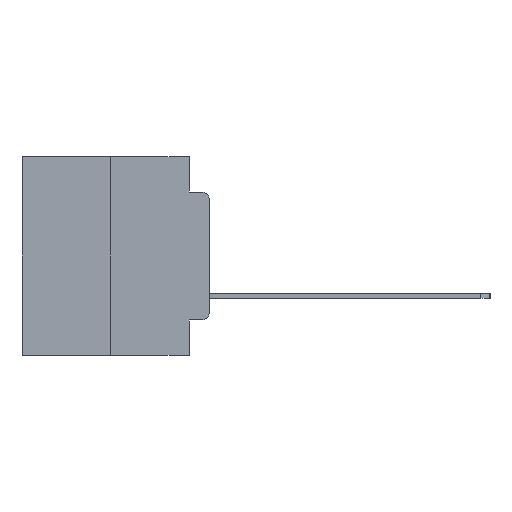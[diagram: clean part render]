
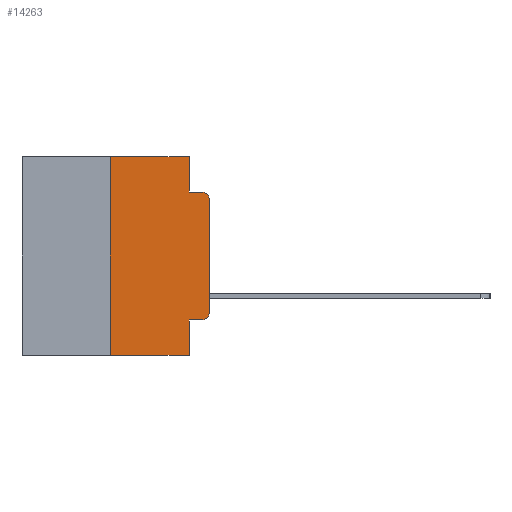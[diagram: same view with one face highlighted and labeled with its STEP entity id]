
A CAD part, left-side view. The second image highlights one B-rep face of the part: STEP entity #14263.
In plain terms, the highlighted planar face has unit normal (-1, 0, 0).
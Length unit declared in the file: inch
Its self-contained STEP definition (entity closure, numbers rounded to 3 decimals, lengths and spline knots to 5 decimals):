
#184 = CARTESIAN_POINT ( 'NONE',  ( 0., 0.051, -0.4115 ) ) ;
#255 = CARTESIAN_POINT ( 'NONE',  ( 0., 0.051, -0.5 ) ) ;
#302 = CARTESIAN_POINT ( 'NONE',  ( 0., 0.25, -0.5 ) ) ;
#664 = VERTEX_POINT ( 'NONE', #302 ) ;
#765 = DIRECTION ( 'NONE',  ( 0., 0., -1. ) ) ;
#1429 = CARTESIAN_POINT ( 'NONE',  ( 0., 0.25, 0. ) ) ;
#1545 = CIRCLE ( 'NONE', #26477, 0.02 ) ;
#1631 = CARTESIAN_POINT ( 'NONE',  ( 0., 0.25, 0. ) ) ;
#1742 = LINE ( 'NONE', #17916, #17604 ) ;
#2095 = VECTOR ( 'NONE', #19553, 39.37008 ) ;
#2428 = PLANE ( 'NONE',  #7140 ) ;
#3873 = CARTESIAN_POINT ( 'NONE',  ( 0., 0.02, -0.1085 ) ) ;
#4136 = VECTOR ( 'NONE', #13969, 39.37008 ) ;
#4396 = VERTEX_POINT ( 'NONE', #21142 ) ;
#4812 = VERTEX_POINT ( 'NONE', #255 ) ;
#5426 = CARTESIAN_POINT ( 'NONE',  ( 0., 0.473, -0.5 ) ) ;
#5463 = DIRECTION ( 'NONE',  ( 0., 0., -1. ) ) ;
#5525 = LINE ( 'NONE', #1429, #4136 ) ;
#6097 = DIRECTION ( 'NONE',  ( 0., 0., -1. ) ) ;
#6150 = VERTEX_POINT ( 'NONE', #8115 ) ;
#6629 = EDGE_CURVE ( 'NONE', #664, #4812, #7875, .T. ) ;
#6829 = DIRECTION ( 'NONE',  ( 0., 0., -1. ) ) ;
#7140 = AXIS2_PLACEMENT_3D ( 'NONE', #16870, #18857, #6829 ) ;
#7439 = EDGE_CURVE ( 'NONE', #664, #12577, #5525, .T. ) ;
#7503 = CARTESIAN_POINT ( 'NONE',  ( 0., 0.051, 0. ) ) ;
#7695 = EDGE_LOOP ( 'NONE', ( #23979, #17189, #19660, #12799, #21220, #23077, #20922, #14076, #24613, #19978 ) ) ;
#7875 = LINE ( 'NONE', #5426, #2095 ) ;
#7946 = EDGE_CURVE ( 'NONE', #4396, #16833, #20316, .T. ) ;
#8115 = CARTESIAN_POINT ( 'NONE',  ( 0., 0.02, -0.4115 ) ) ;
#8444 = DIRECTION ( 'NONE',  ( 0., -1., 0. ) ) ;
#8752 = VECTOR ( 'NONE', #16467, 39.37008 ) ;
#8788 = EDGE_CURVE ( 'NONE', #13639, #4812, #17492, .T. ) ;
#10170 = CARTESIAN_POINT ( 'NONE',  ( 0., 0., -0.1085 ) ) ;
#10234 = LINE ( 'NONE', #12198, #24893 ) ;
#10654 = EDGE_CURVE ( 'NONE', #6150, #22400, #1545, .T. ) ;
#11396 = CARTESIAN_POINT ( 'NONE',  ( 0., 0.051, 0. ) ) ;
#11685 = CARTESIAN_POINT ( 'NONE',  ( 0., 0.02, -0.3915 ) ) ;
#12155 = CARTESIAN_POINT ( 'NONE',  ( 0., 0., -0.3915 ) ) ;
#12156 = VECTOR ( 'NONE', #5463, 39.37008 ) ;
#12170 = VERTEX_POINT ( 'NONE', #12856 ) ;
#12198 = CARTESIAN_POINT ( 'NONE',  ( 0., 0., 0. ) ) ;
#12577 = VERTEX_POINT ( 'NONE', #1631 ) ;
#12799 = ORIENTED_EDGE ( 'NONE', *, *, #7946, .F. ) ;
#12856 = CARTESIAN_POINT ( 'NONE',  ( 0., 0.02, -0.0885 ) ) ;
#13639 = VERTEX_POINT ( 'NONE', #184 ) ;
#13710 = DIRECTION ( 'NONE',  ( 0., 0., -1. ) ) ;
#13969 = DIRECTION ( 'NONE',  ( 0., 0., 1. ) ) ;
#14076 = ORIENTED_EDGE ( 'NONE', *, *, #8788, .F. ) ;
#14212 = DIRECTION ( 'NONE',  ( 0., 0., 1. ) ) ;
#14263 = ADVANCED_FACE ( 'NONE', ( #15084 ), #2428, .F. ) ;
#14432 = CARTESIAN_POINT ( 'NONE',  ( 0., 0.051, -0.0885 ) ) ;
#14462 = AXIS2_PLACEMENT_3D ( 'NONE', #3873, #18154, #6097 ) ;
#15084 = FACE_OUTER_BOUND ( 'NONE', #7695, .T. ) ;
#16467 = DIRECTION ( 'NONE',  ( 0., -1., 0. ) ) ;
#16529 = EDGE_CURVE ( 'NONE', #22400, #16530, #10234, .T. ) ;
#16530 = VERTEX_POINT ( 'NONE', #10170 ) ;
#16833 = VERTEX_POINT ( 'NONE', #17115 ) ;
#16870 = CARTESIAN_POINT ( 'NONE',  ( 0., 0.473, 0. ) ) ;
#17115 = CARTESIAN_POINT ( 'NONE',  ( 0., 0.051, -0.0885 ) ) ;
#17189 = ORIENTED_EDGE ( 'NONE', *, *, #19177, .T. ) ;
#17492 = LINE ( 'NONE', #7503, #12156 ) ;
#17604 = VECTOR ( 'NONE', #19918, 39.37008 ) ;
#17916 = CARTESIAN_POINT ( 'NONE',  ( 0., 0.051, -0.4115 ) ) ;
#18154 = DIRECTION ( 'NONE',  ( -1., 0., 0. ) ) ;
#18857 = DIRECTION ( 'NONE',  ( 1., 0., 0. ) ) ;
#19177 = EDGE_CURVE ( 'NONE', #16530, #12170, #24083, .T. ) ;
#19525 = EDGE_CURVE ( 'NONE', #13639, #6150, #1742, .T. ) ;
#19553 = DIRECTION ( 'NONE',  ( 0., -1., 0. ) ) ;
#19631 = VECTOR ( 'NONE', #8444, 39.37008 ) ;
#19660 = ORIENTED_EDGE ( 'NONE', *, *, #24483, .F. ) ;
#19729 = EDGE_CURVE ( 'NONE', #12577, #4396, #24404, .T. ) ;
#19918 = DIRECTION ( 'NONE',  ( 0., -1., 0. ) ) ;
#19978 = ORIENTED_EDGE ( 'NONE', *, *, #10654, .T. ) ;
#20316 = LINE ( 'NONE', #11396, #25611 ) ;
#20922 = ORIENTED_EDGE ( 'NONE', *, *, #6629, .T. ) ;
#21142 = CARTESIAN_POINT ( 'NONE',  ( 0., 0.051, 0. ) ) ;
#21220 = ORIENTED_EDGE ( 'NONE', *, *, #19729, .F. ) ;
#22400 = VERTEX_POINT ( 'NONE', #12155 ) ;
#22401 = CARTESIAN_POINT ( 'NONE',  ( 0., 0.473, 0. ) ) ;
#23077 = ORIENTED_EDGE ( 'NONE', *, *, #7439, .F. ) ;
#23979 = ORIENTED_EDGE ( 'NONE', *, *, #16529, .T. ) ;
#24083 = CIRCLE ( 'NONE', #14462, 0.02 ) ;
#24404 = LINE ( 'NONE', #22401, #19631 ) ;
#24483 = EDGE_CURVE ( 'NONE', #16833, #12170, #24649, .T. ) ;
#24613 = ORIENTED_EDGE ( 'NONE', *, *, #19525, .T. ) ;
#24649 = LINE ( 'NONE', #14432, #8752 ) ;
#24893 = VECTOR ( 'NONE', #14212, 39.37008 ) ;
#25611 = VECTOR ( 'NONE', #765, 39.37008 ) ;
#25637 = DIRECTION ( 'NONE',  ( -1., 0., 0. ) ) ;
#26477 = AXIS2_PLACEMENT_3D ( 'NONE', #11685, #25637, #13710 ) ;
